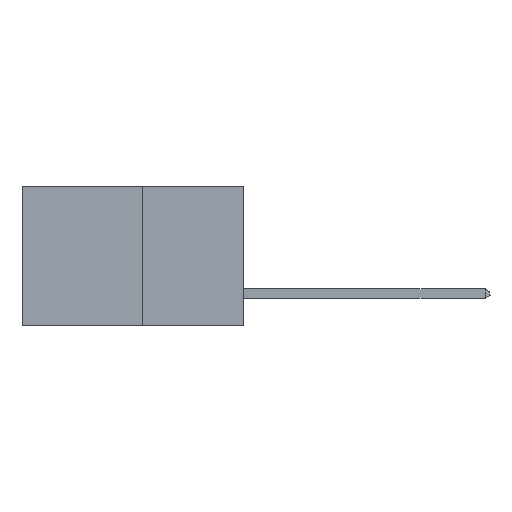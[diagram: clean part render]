
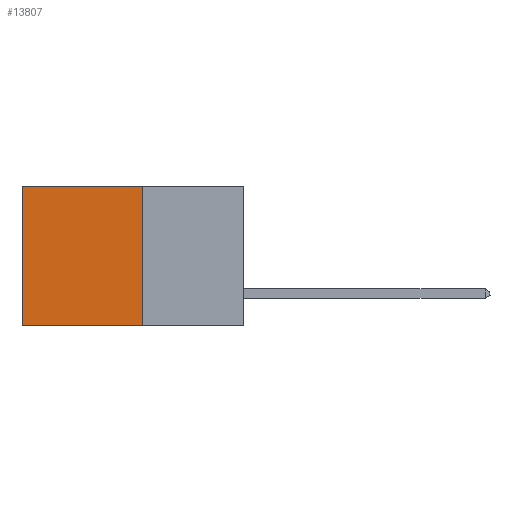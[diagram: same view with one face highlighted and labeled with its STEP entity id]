
A CAD part, left-side view. The second image highlights one B-rep face of the part: STEP entity #13807.
In plain terms, the highlighted planar face has unit normal (-1, 0, 0).
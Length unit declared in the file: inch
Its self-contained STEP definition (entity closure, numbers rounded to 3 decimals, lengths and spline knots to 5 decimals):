
#124 = CARTESIAN_POINT ( 'NONE',  ( 0.277, 0.27, -0.37 ) ) ;
#839 = LINE ( 'NONE', #16806, #15751 ) ;
#893 = LINE ( 'NONE', #12572, #4934 ) ;
#1258 = CARTESIAN_POINT ( 'NONE',  ( 0.277, 0.59, -0.37 ) ) ;
#1444 = EDGE_CURVE ( 'NONE', #3074, #12940, #893, .T. ) ;
#1537 = FACE_OUTER_BOUND ( 'NONE', #2053, .T. ) ;
#1838 = ORIENTED_EDGE ( 'NONE', *, *, #3729, .T. ) ;
#2053 = EDGE_LOOP ( 'NONE', ( #8065, #15381, #16223, #1838 ) ) ;
#2253 = LINE ( 'NONE', #11567, #13347 ) ;
#2880 = EDGE_CURVE ( 'NONE', #3549, #3074, #839, .T. ) ;
#3074 = VERTEX_POINT ( 'NONE', #8844 ) ;
#3246 = DIRECTION ( 'NONE',  ( 0., 0., -1. ) ) ;
#3549 = VERTEX_POINT ( 'NONE', #15357 ) ;
#3729 = EDGE_CURVE ( 'NONE', #3549, #10010, #2253, .T. ) ;
#3764 = CARTESIAN_POINT ( 'NONE',  ( 0.277, 0.59, 0. ) ) ;
#4336 = DIRECTION ( 'NONE',  ( 0., 1., 0. ) ) ;
#4934 = VECTOR ( 'NONE', #12546, 39.37008 ) ;
#5274 = CARTESIAN_POINT ( 'NONE',  ( 0.277, 0.59, -0.37 ) ) ;
#7001 = DIRECTION ( 'NONE',  ( 0., 0., -1. ) ) ;
#8065 = ORIENTED_EDGE ( 'NONE', *, *, #14747, .T. ) ;
#8145 = DIRECTION ( 'NONE',  ( 0., 0., -1. ) ) ;
#8844 = CARTESIAN_POINT ( 'NONE',  ( 0.277, 0.27, -0.37 ) ) ;
#9092 = PLANE ( 'NONE',  #16726 ) ;
#10010 = VERTEX_POINT ( 'NONE', #3764 ) ;
#10518 = VECTOR ( 'NONE', #8145, 39.37008 ) ;
#11567 = CARTESIAN_POINT ( 'NONE',  ( 0.277, 0.27, 0. ) ) ;
#11942 = DIRECTION ( 'NONE',  ( 1., 0., 0. ) ) ;
#12546 = DIRECTION ( 'NONE',  ( 0., 1., 0. ) ) ;
#12572 = CARTESIAN_POINT ( 'NONE',  ( 0.277, 0.27, -0.37 ) ) ;
#12940 = VERTEX_POINT ( 'NONE', #1258 ) ;
#13347 = VECTOR ( 'NONE', #4336, 39.37008 ) ;
#13807 = ADVANCED_FACE ( 'NONE', ( #1537 ), #9092, .F. ) ;
#14205 = LINE ( 'NONE', #5274, #10518 ) ;
#14747 = EDGE_CURVE ( 'NONE', #10010, #12940, #14205, .T. ) ;
#15357 = CARTESIAN_POINT ( 'NONE',  ( 0.277, 0.27, 0. ) ) ;
#15381 = ORIENTED_EDGE ( 'NONE', *, *, #1444, .F. ) ;
#15751 = VECTOR ( 'NONE', #7001, 39.37008 ) ;
#16223 = ORIENTED_EDGE ( 'NONE', *, *, #2880, .F. ) ;
#16726 = AXIS2_PLACEMENT_3D ( 'NONE', #124, #11942, #3246 ) ;
#16806 = CARTESIAN_POINT ( 'NONE',  ( 0.277, 0.27, -0.37 ) ) ;
